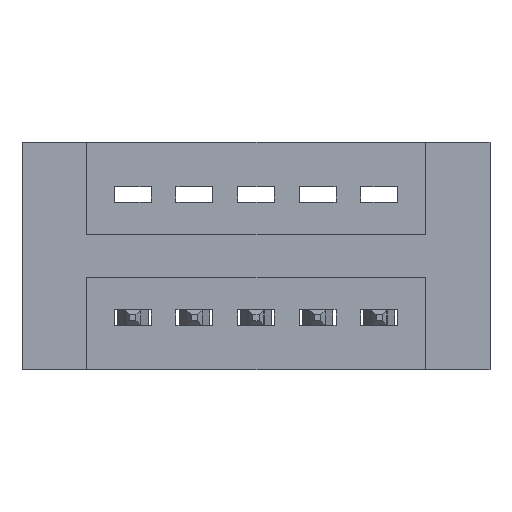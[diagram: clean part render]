
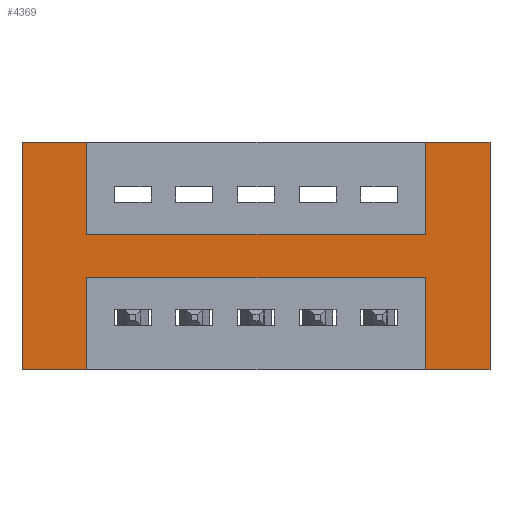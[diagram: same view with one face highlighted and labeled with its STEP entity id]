
A CAD part, front view. The second image highlights one B-rep face of the part: STEP entity #4369.
In plain terms, the highlighted planar face has unit normal (0, -1, 0).
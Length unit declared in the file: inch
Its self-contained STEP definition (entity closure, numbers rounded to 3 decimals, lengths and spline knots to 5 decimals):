
#55 = CARTESIAN_POINT ( 'NONE',  ( 0.9425, 0., -0.22 ) ) ;
#200 = VECTOR ( 'NONE', #7206, 39.37008 ) ;
#223 = VERTEX_POINT ( 'NONE', #55 ) ;
#229 = CARTESIAN_POINT ( 'NONE',  ( 0.9425, 0., 0. ) ) ;
#310 = CARTESIAN_POINT ( 'NONE',  ( 0.3925, 0., 0. ) ) ;
#335 = EDGE_LOOP ( 'NONE', ( #7381, #1620, #2004, #2023, #2151, #4265, #3332, #4561, #4993, #7004, #4546, #6006 ) ) ;
#416 = CARTESIAN_POINT ( 'NONE',  ( 0., 0., -0.37 ) ) ;
#614 = CARTESIAN_POINT ( 'NONE',  ( 0.9425, 0., -0.37 ) ) ;
#635 = VECTOR ( 'NONE', #6021, 39.37008 ) ;
#727 = EDGE_CURVE ( 'NONE', #3310, #4440, #4514, .T. ) ;
#952 = CARTESIAN_POINT ( 'NONE',  ( 0.2875, 0., -0.37 ) ) ;
#1000 = LINE ( 'NONE', #4722, #5794 ) ;
#1213 = CARTESIAN_POINT ( 'NONE',  ( 0.9425, 0., 0. ) ) ;
#1256 = DIRECTION ( 'NONE',  ( 0., 0., 1. ) ) ;
#1350 = CARTESIAN_POINT ( 'NONE',  ( 0.3925, 0., -0.15 ) ) ;
#1409 = CARTESIAN_POINT ( 'NONE',  ( 0., 0., 0. ) ) ;
#1532 = LINE ( 'NONE', #1409, #635 ) ;
#1600 = VECTOR ( 'NONE', #5089, 39.37008 ) ;
#1620 = ORIENTED_EDGE ( 'NONE', *, *, #6875, .F. ) ;
#1649 = LINE ( 'NONE', #4370, #4099 ) ;
#1942 = LINE ( 'NONE', #6059, #6449 ) ;
#1964 = CARTESIAN_POINT ( 'NONE',  ( 1.0475, 0., -0.37 ) ) ;
#1989 = EDGE_CURVE ( 'NONE', #4440, #8443, #8460, .T. ) ;
#2004 = ORIENTED_EDGE ( 'NONE', *, *, #1989, .F. ) ;
#2013 = EDGE_CURVE ( 'NONE', #5430, #3552, #6702, .T. ) ;
#2023 = ORIENTED_EDGE ( 'NONE', *, *, #727, .F. ) ;
#2151 = ORIENTED_EDGE ( 'NONE', *, *, #4462, .F. ) ;
#2358 = PLANE ( 'NONE',  #5683 ) ;
#2375 = CARTESIAN_POINT ( 'NONE',  ( 0.3925, 0., -0.15 ) ) ;
#2380 = VERTEX_POINT ( 'NONE', #2609 ) ;
#2407 = EDGE_CURVE ( 'NONE', #223, #3822, #7326, .T. ) ;
#2609 = CARTESIAN_POINT ( 'NONE',  ( 0.2875, 0., 0. ) ) ;
#2887 = DIRECTION ( 'NONE',  ( -1., 0., 0. ) ) ;
#2968 = CARTESIAN_POINT ( 'NONE',  ( 0., 0., 0. ) ) ;
#3310 = VERTEX_POINT ( 'NONE', #2375 ) ;
#3332 = ORIENTED_EDGE ( 'NONE', *, *, #7237, .T. ) ;
#3333 = LINE ( 'NONE', #7896, #1600 ) ;
#3434 = VECTOR ( 'NONE', #7412, 39.37008 ) ;
#3552 = VERTEX_POINT ( 'NONE', #4016 ) ;
#3822 = VERTEX_POINT ( 'NONE', #6508 ) ;
#4016 = CARTESIAN_POINT ( 'NONE',  ( 1.0475, 0., 0. ) ) ;
#4099 = VECTOR ( 'NONE', #6359, 39.37008 ) ;
#4120 = EDGE_CURVE ( 'NONE', #5430, #6742, #1649, .T. ) ;
#4147 = CARTESIAN_POINT ( 'NONE',  ( 0.9425, 0., -0.15 ) ) ;
#4265 = ORIENTED_EDGE ( 'NONE', *, *, #7537, .F. ) ;
#4369 = ADVANCED_FACE ( 'NONE', ( #4513 ), #2358, .T. ) ;
#4370 = CARTESIAN_POINT ( 'NONE',  ( 0., 0., -0.37 ) ) ;
#4440 = VERTEX_POINT ( 'NONE', #4147 ) ;
#4462 = EDGE_CURVE ( 'NONE', #5122, #3310, #1942, .T. ) ;
#4513 = FACE_OUTER_BOUND ( 'NONE', #335, .T. ) ;
#4514 = LINE ( 'NONE', #1350, #200 ) ;
#4546 = ORIENTED_EDGE ( 'NONE', *, *, #6696, .F. ) ;
#4561 = ORIENTED_EDGE ( 'NONE', *, *, #7174, .F. ) ;
#4667 = DIRECTION ( 'NONE',  ( 0., 0., -1. ) ) ;
#4722 = CARTESIAN_POINT ( 'NONE',  ( 0., 0., -0.37 ) ) ;
#4748 = LINE ( 'NONE', #4761, #5365 ) ;
#4761 = CARTESIAN_POINT ( 'NONE',  ( 0.3925, 0., -0.37 ) ) ;
#4819 = VERTEX_POINT ( 'NONE', #952 ) ;
#4967 = DIRECTION ( 'NONE',  ( 0., 0., -1. ) ) ;
#4993 = ORIENTED_EDGE ( 'NONE', *, *, #8373, .F. ) ;
#5089 = DIRECTION ( 'NONE',  ( 0., 0., -1. ) ) ;
#5122 = VERTEX_POINT ( 'NONE', #310 ) ;
#5365 = VECTOR ( 'NONE', #4667, 39.37008 ) ;
#5430 = VERTEX_POINT ( 'NONE', #1964 ) ;
#5567 = DIRECTION ( 'NONE',  ( -1., 0., 0. ) ) ;
#5683 = AXIS2_PLACEMENT_3D ( 'NONE', #416, #8243, #4967 ) ;
#5778 = VECTOR ( 'NONE', #5567, 39.37008 ) ;
#5794 = VECTOR ( 'NONE', #2887, 39.37008 ) ;
#6006 = ORIENTED_EDGE ( 'NONE', *, *, #4120, .F. ) ;
#6021 = DIRECTION ( 'NONE',  ( 1., 0., 0. ) ) ;
#6059 = CARTESIAN_POINT ( 'NONE',  ( 0.3925, 0., 0. ) ) ;
#6093 = DIRECTION ( 'NONE',  ( 0., 0., -1. ) ) ;
#6334 = CARTESIAN_POINT ( 'NONE',  ( 0.9425, 0., -0.37 ) ) ;
#6359 = DIRECTION ( 'NONE',  ( -1., 0., 0. ) ) ;
#6449 = VECTOR ( 'NONE', #6093, 39.37008 ) ;
#6508 = CARTESIAN_POINT ( 'NONE',  ( 0.3925, 0., -0.22 ) ) ;
#6593 = VECTOR ( 'NONE', #7804, 39.37008 ) ;
#6696 = EDGE_CURVE ( 'NONE', #6742, #223, #7692, .T. ) ;
#6702 = LINE ( 'NONE', #7379, #3434 ) ;
#6742 = VERTEX_POINT ( 'NONE', #6334 ) ;
#6851 = CARTESIAN_POINT ( 'NONE',  ( 0.3925, 0., -0.37 ) ) ;
#6875 = EDGE_CURVE ( 'NONE', #8443, #3552, #1532, .T. ) ;
#7004 = ORIENTED_EDGE ( 'NONE', *, *, #2407, .F. ) ;
#7174 = EDGE_CURVE ( 'NONE', #8501, #4819, #1000, .T. ) ;
#7206 = DIRECTION ( 'NONE',  ( 1., 0., 0. ) ) ;
#7237 = EDGE_CURVE ( 'NONE', #2380, #4819, #3333, .T. ) ;
#7326 = LINE ( 'NONE', #7472, #5778 ) ;
#7379 = CARTESIAN_POINT ( 'NONE',  ( 1.0475, 0., 0. ) ) ;
#7381 = ORIENTED_EDGE ( 'NONE', *, *, #2013, .T. ) ;
#7412 = DIRECTION ( 'NONE',  ( 0., 0., 1. ) ) ;
#7472 = CARTESIAN_POINT ( 'NONE',  ( 0.3925, 0., -0.22 ) ) ;
#7487 = DIRECTION ( 'NONE',  ( 1., 0., 0. ) ) ;
#7537 = EDGE_CURVE ( 'NONE', #2380, #5122, #7562, .T. ) ;
#7562 = LINE ( 'NONE', #2968, #8163 ) ;
#7692 = LINE ( 'NONE', #614, #8171 ) ;
#7804 = DIRECTION ( 'NONE',  ( 0., 0., 1. ) ) ;
#7896 = CARTESIAN_POINT ( 'NONE',  ( 0.2875, 0., 0. ) ) ;
#8163 = VECTOR ( 'NONE', #7487, 39.37008 ) ;
#8171 = VECTOR ( 'NONE', #1256, 39.37008 ) ;
#8243 = DIRECTION ( 'NONE',  ( 0., -1., 0. ) ) ;
#8373 = EDGE_CURVE ( 'NONE', #3822, #8501, #4748, .T. ) ;
#8443 = VERTEX_POINT ( 'NONE', #229 ) ;
#8460 = LINE ( 'NONE', #1213, #6593 ) ;
#8501 = VERTEX_POINT ( 'NONE', #6851 ) ;
